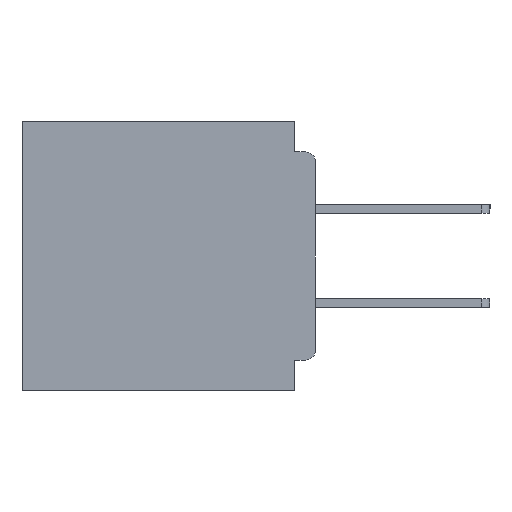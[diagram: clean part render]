
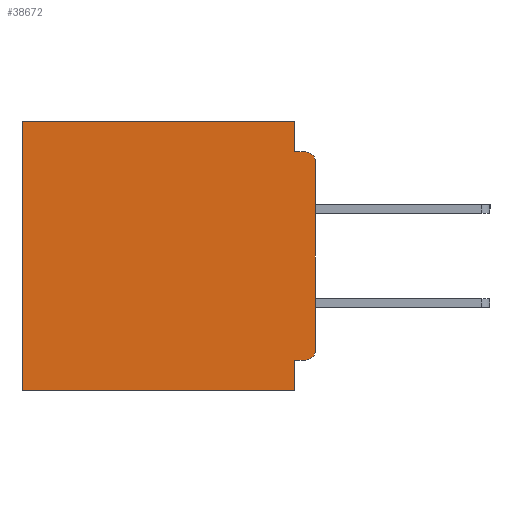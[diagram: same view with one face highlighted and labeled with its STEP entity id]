
A CAD part, left-side view. The second image highlights one B-rep face of the part: STEP entity #38672.
In plain terms, the highlighted planar face has unit normal (-1, 0, 0).
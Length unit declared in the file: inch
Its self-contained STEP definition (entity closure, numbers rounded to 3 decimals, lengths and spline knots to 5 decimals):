
#1131 = VECTOR ( 'NONE', #30793, 39.37008 ) ;
#1393 = CARTESIAN_POINT ( 'NONE',  ( 0.3, 0.031, -0.4 ) ) ;
#1767 = AXIS2_PLACEMENT_3D ( 'NONE', #14249, #47922, #19090 ) ;
#2486 = ORIENTED_EDGE ( 'NONE', *, *, #50236, .T. ) ;
#2702 = VECTOR ( 'NONE', #19427, 39.37008 ) ;
#2893 = ORIENTED_EDGE ( 'NONE', *, *, #17898, .F. ) ;
#3926 = CARTESIAN_POINT ( 'NONE',  ( 0.3, 0.015, -0.34 ) ) ;
#5828 = VERTEX_POINT ( 'NONE', #17745 ) ;
#7729 = CARTESIAN_POINT ( 'NONE',  ( 0.3, 0.031, -0.355 ) ) ;
#7865 = DIRECTION ( 'NONE',  ( 0., 0., -1. ) ) ;
#7985 = LINE ( 'NONE', #28073, #43409 ) ;
#8466 = VECTOR ( 'NONE', #32985, 39.37008 ) ;
#8807 = ORIENTED_EDGE ( 'NONE', *, *, #25236, .F. ) ;
#8848 = DIRECTION ( 'NONE',  ( 0., 0., -1. ) ) ;
#10341 = CARTESIAN_POINT ( 'NONE',  ( 0.3, 0.437, -0.4 ) ) ;
#10772 = LINE ( 'NONE', #53857, #36415 ) ;
#14073 = LINE ( 'NONE', #16260, #1131 ) ;
#14249 = CARTESIAN_POINT ( 'NONE',  ( 0.3, 0., -0.4 ) ) ;
#14856 = ORIENTED_EDGE ( 'NONE', *, *, #55298, .T. ) ;
#15363 = DIRECTION ( 'NONE',  ( 0., 0., -1. ) ) ;
#15673 = AXIS2_PLACEMENT_3D ( 'NONE', #50009, #21167, #54865 ) ;
#16260 = CARTESIAN_POINT ( 'NONE',  ( 0.3, 0., -0.4 ) ) ;
#17135 = VECTOR ( 'NONE', #7865, 39.37008 ) ;
#17745 = CARTESIAN_POINT ( 'NONE',  ( 0.3, 0.015, -0.045 ) ) ;
#17898 = EDGE_CURVE ( 'NONE', #41258, #19179, #14073, .T. ) ;
#19090 = DIRECTION ( 'NONE',  ( 0., 0., -1. ) ) ;
#19179 = VERTEX_POINT ( 'NONE', #40291 ) ;
#19256 = VERTEX_POINT ( 'NONE', #45756 ) ;
#19427 = DIRECTION ( 'NONE',  ( 0., -1., 0. ) ) ;
#20416 = EDGE_CURVE ( 'NONE', #39363, #5828, #22102, .T. ) ;
#20473 = VECTOR ( 'NONE', #29522, 39.37008 ) ;
#21167 = DIRECTION ( 'NONE',  ( -1., 0., 0. ) ) ;
#21867 = VERTEX_POINT ( 'NONE', #35629 ) ;
#22102 = CIRCLE ( 'NONE', #15673, 0.015 ) ;
#24063 = EDGE_CURVE ( 'NONE', #19256, #45365, #38391, .T. ) ;
#24601 = VERTEX_POINT ( 'NONE', #7729 ) ;
#25236 = EDGE_CURVE ( 'NONE', #39363, #45365, #29953, .T. ) ;
#27307 = FACE_OUTER_BOUND ( 'NONE', #28006, .T. ) ;
#28006 = EDGE_LOOP ( 'NONE', ( #8807, #45342, #48804, #29450, #2486, #14856, #2893, #44530, #48628, #53365 ) ) ;
#28073 = CARTESIAN_POINT ( 'NONE',  ( 0.3, 0.031, 0. ) ) ;
#28195 = LINE ( 'NONE', #55178, #39502 ) ;
#28434 = LINE ( 'NONE', #48251, #2702 ) ;
#28686 = CARTESIAN_POINT ( 'NONE',  ( 0.3, 0., -0.06 ) ) ;
#29450 = ORIENTED_EDGE ( 'NONE', *, *, #61305, .F. ) ;
#29522 = DIRECTION ( 'NONE',  ( 0., 0., -1. ) ) ;
#29743 = AXIS2_PLACEMENT_3D ( 'NONE', #3926, #37720, #8848 ) ;
#29953 = LINE ( 'NONE', #51026, #17135 ) ;
#30793 = DIRECTION ( 'NONE',  ( 0., 1., 0. ) ) ;
#32985 = DIRECTION ( 'NONE',  ( 0., 1., 0. ) ) ;
#33976 = EDGE_CURVE ( 'NONE', #24601, #41258, #10772, .T. ) ;
#34862 = LINE ( 'NONE', #10341, #20473 ) ;
#34891 = EDGE_CURVE ( 'NONE', #19256, #24601, #59624, .T. ) ;
#35629 = CARTESIAN_POINT ( 'NONE',  ( 0.3, 0.031, 0. ) ) ;
#36415 = VECTOR ( 'NONE', #15363, 39.37008 ) ;
#37720 = DIRECTION ( 'NONE',  ( -1., 0., 0. ) ) ;
#38260 = PLANE ( 'NONE',  #1767 ) ;
#38391 = CIRCLE ( 'NONE', #29743, 0.015 ) ;
#38672 = ADVANCED_FACE ( 'NONE', ( #27307 ), #38260, .F. ) ;
#39363 = VERTEX_POINT ( 'NONE', #28686 ) ;
#39502 = VECTOR ( 'NONE', #50300, 39.37008 ) ;
#40291 = CARTESIAN_POINT ( 'NONE',  ( 0.3, 0.437, -0.4 ) ) ;
#41089 = CARTESIAN_POINT ( 'NONE',  ( 0.3, 0.031, -0.045 ) ) ;
#41258 = VERTEX_POINT ( 'NONE', #1393 ) ;
#41406 = VERTEX_POINT ( 'NONE', #41089 ) ;
#42589 = DIRECTION ( 'NONE',  ( 0., 0., -1. ) ) ;
#42934 = CARTESIAN_POINT ( 'NONE',  ( 0.3, 0.437, 0. ) ) ;
#43409 = VECTOR ( 'NONE', #42589, 39.37008 ) ;
#44530 = ORIENTED_EDGE ( 'NONE', *, *, #33976, .F. ) ;
#45342 = ORIENTED_EDGE ( 'NONE', *, *, #20416, .T. ) ;
#45365 = VERTEX_POINT ( 'NONE', #54098 ) ;
#45756 = CARTESIAN_POINT ( 'NONE',  ( 0.3, 0.015, -0.355 ) ) ;
#47922 = DIRECTION ( 'NONE',  ( 1., 0., 0. ) ) ;
#48251 = CARTESIAN_POINT ( 'NONE',  ( 0.3, 0., -0.045 ) ) ;
#48487 = EDGE_CURVE ( 'NONE', #41406, #5828, #28434, .T. ) ;
#48628 = ORIENTED_EDGE ( 'NONE', *, *, #34891, .F. ) ;
#48804 = ORIENTED_EDGE ( 'NONE', *, *, #48487, .F. ) ;
#50009 = CARTESIAN_POINT ( 'NONE',  ( 0.3, 0.015, -0.06 ) ) ;
#50236 = EDGE_CURVE ( 'NONE', #21867, #55720, #28195, .T. ) ;
#50300 = DIRECTION ( 'NONE',  ( 0., 1., 0. ) ) ;
#51026 = CARTESIAN_POINT ( 'NONE',  ( 0.3, 0., -0.4 ) ) ;
#53365 = ORIENTED_EDGE ( 'NONE', *, *, #24063, .T. ) ;
#53857 = CARTESIAN_POINT ( 'NONE',  ( 0.3, 0.031, -0.4 ) ) ;
#54098 = CARTESIAN_POINT ( 'NONE',  ( 0.3, 0., -0.34 ) ) ;
#54865 = DIRECTION ( 'NONE',  ( 0., 0., -1. ) ) ;
#55178 = CARTESIAN_POINT ( 'NONE',  ( 0.3, 0., 0. ) ) ;
#55298 = EDGE_CURVE ( 'NONE', #55720, #19179, #34862, .T. ) ;
#55720 = VERTEX_POINT ( 'NONE', #42934 ) ;
#56875 = CARTESIAN_POINT ( 'NONE',  ( 0.3, 0., -0.355 ) ) ;
#59624 = LINE ( 'NONE', #56875, #8466 ) ;
#61305 = EDGE_CURVE ( 'NONE', #21867, #41406, #7985, .T. ) ;
